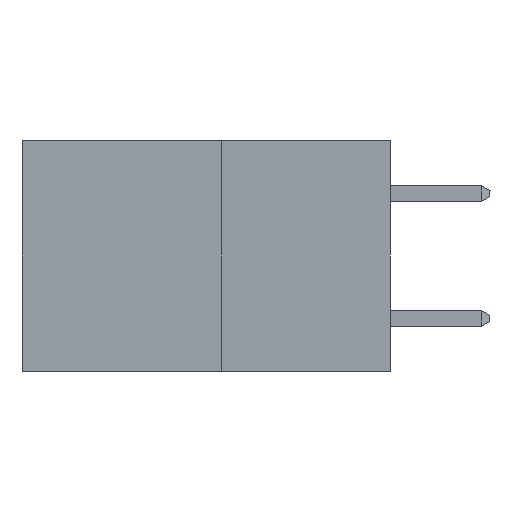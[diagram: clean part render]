
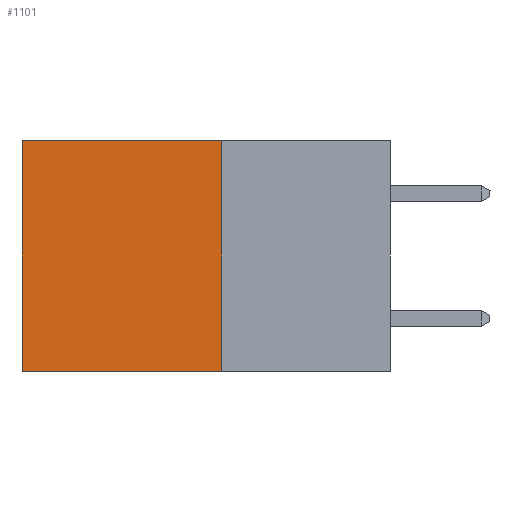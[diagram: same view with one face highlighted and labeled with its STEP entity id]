
A CAD part, left-side view. The second image highlights one B-rep face of the part: STEP entity #1101.
In plain terms, the highlighted planar face has unit normal (-1, 0, 0).
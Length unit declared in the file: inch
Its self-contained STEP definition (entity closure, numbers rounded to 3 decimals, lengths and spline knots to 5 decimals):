
#175 = VERTEX_POINT ( 'NONE', #3456 ) ;
#736 = EDGE_CURVE ( 'NONE', #4390, #8830, #3603, .T. ) ;
#746 = DIRECTION ( 'NONE',  ( 0., 1., 0. ) ) ;
#770 = CARTESIAN_POINT ( 'NONE',  ( 0.277, 0.27, -0.37 ) ) ;
#878 = FACE_OUTER_BOUND ( 'NONE', #6961, .T. ) ;
#1012 = ORIENTED_EDGE ( 'NONE', *, *, #7718, .T. ) ;
#1024 = PLANE ( 'NONE',  #9480 ) ;
#1101 = ADVANCED_FACE ( 'NONE', ( #878 ), #1024, .F. ) ;
#1294 = ORIENTED_EDGE ( 'NONE', *, *, #736, .F. ) ;
#1794 = CARTESIAN_POINT ( 'NONE',  ( 0.277, 0.27, 0. ) ) ;
#2246 = LINE ( 'NONE', #1794, #10941 ) ;
#2325 = VECTOR ( 'NONE', #746, 39.37008 ) ;
#2797 = VERTEX_POINT ( 'NONE', #10832 ) ;
#2931 = EDGE_CURVE ( 'NONE', #4390, #2797, #2246, .T. ) ;
#2944 = CARTESIAN_POINT ( 'NONE',  ( 0.277, 0.27, -0.37 ) ) ;
#3456 = CARTESIAN_POINT ( 'NONE',  ( 0.277, 0.59, -0.37 ) ) ;
#3533 = LINE ( 'NONE', #4861, #9948 ) ;
#3603 = LINE ( 'NONE', #10711, #7310 ) ;
#3726 = ORIENTED_EDGE ( 'NONE', *, *, #2931, .T. ) ;
#4270 = DIRECTION ( 'NONE',  ( 0., 0., -1. ) ) ;
#4390 = VERTEX_POINT ( 'NONE', #5811 ) ;
#4631 = DIRECTION ( 'NONE',  ( 0., 0., -1. ) ) ;
#4861 = CARTESIAN_POINT ( 'NONE',  ( 0.277, 0.59, -0.37 ) ) ;
#5811 = CARTESIAN_POINT ( 'NONE',  ( 0.277, 0.27, 0. ) ) ;
#6961 = EDGE_LOOP ( 'NONE', ( #1012, #7953, #1294, #3726 ) ) ;
#7201 = LINE ( 'NONE', #770, #2325 ) ;
#7310 = VECTOR ( 'NONE', #10637, 39.37008 ) ;
#7718 = EDGE_CURVE ( 'NONE', #2797, #175, #3533, .T. ) ;
#7953 = ORIENTED_EDGE ( 'NONE', *, *, #10781, .F. ) ;
#8209 = CARTESIAN_POINT ( 'NONE',  ( 0.277, 0.27, -0.37 ) ) ;
#8830 = VERTEX_POINT ( 'NONE', #8209 ) ;
#9077 = DIRECTION ( 'NONE',  ( 1., 0., 0. ) ) ;
#9129 = DIRECTION ( 'NONE',  ( 0., 1., 0. ) ) ;
#9480 = AXIS2_PLACEMENT_3D ( 'NONE', #2944, #9077, #4270 ) ;
#9948 = VECTOR ( 'NONE', #4631, 39.37008 ) ;
#10637 = DIRECTION ( 'NONE',  ( 0., 0., -1. ) ) ;
#10711 = CARTESIAN_POINT ( 'NONE',  ( 0.277, 0.27, -0.37 ) ) ;
#10781 = EDGE_CURVE ( 'NONE', #8830, #175, #7201, .T. ) ;
#10832 = CARTESIAN_POINT ( 'NONE',  ( 0.277, 0.59, 0. ) ) ;
#10941 = VECTOR ( 'NONE', #9129, 39.37008 ) ;
